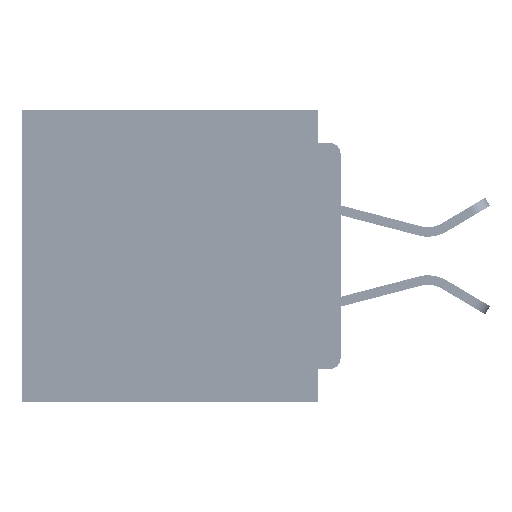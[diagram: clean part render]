
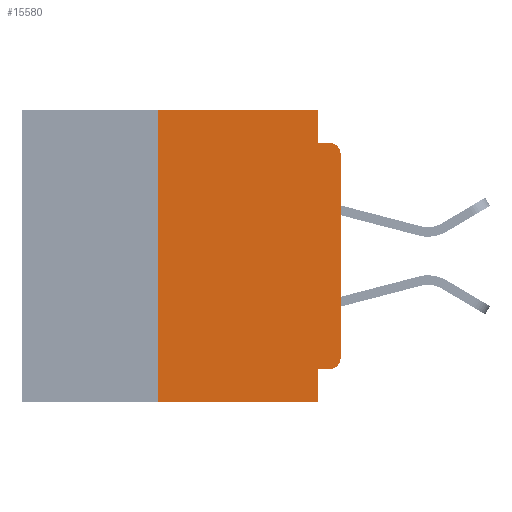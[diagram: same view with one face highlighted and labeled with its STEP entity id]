
A CAD part, left-side view. The second image highlights one B-rep face of the part: STEP entity #15580.
In plain terms, the highlighted planar face has unit normal (-1, 0, 0).
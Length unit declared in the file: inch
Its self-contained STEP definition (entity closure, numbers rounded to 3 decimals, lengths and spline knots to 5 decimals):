
#368 = LINE ( 'NONE', #5651, #32246 ) ;
#454 = ORIENTED_EDGE ( 'NONE', *, *, #24105, .F. ) ;
#1129 = VECTOR ( 'NONE', #30688, 39.37008 ) ;
#1462 = DIRECTION ( 'NONE',  ( 0., 0., 1. ) ) ;
#2603 = VERTEX_POINT ( 'NONE', #30945 ) ;
#2815 = DIRECTION ( 'NONE',  ( -1., 0., 0. ) ) ;
#2857 = CARTESIAN_POINT ( 'NONE',  ( 0., 0.031, -0.4 ) ) ;
#4111 = CARTESIAN_POINT ( 'NONE',  ( 0., 0.015, -0.34 ) ) ;
#5029 = VECTOR ( 'NONE', #46792, 39.37008 ) ;
#5651 = CARTESIAN_POINT ( 'NONE',  ( 0., 0.25, -0.4 ) ) ;
#6347 = AXIS2_PLACEMENT_3D ( 'NONE', #6583, #43711, #19190 ) ;
#6428 = VECTOR ( 'NONE', #40289, 39.37008 ) ;
#6542 = CIRCLE ( 'NONE', #32352, 0.015 ) ;
#6583 = CARTESIAN_POINT ( 'NONE',  ( 0., 0.437, 0. ) ) ;
#6771 = EDGE_CURVE ( 'NONE', #16942, #22062, #12229, .T. ) ;
#7743 = LINE ( 'NONE', #36195, #6428 ) ;
#8335 = DIRECTION ( 'NONE',  ( 0., 0., -1. ) ) ;
#8423 = VECTOR ( 'NONE', #39313, 39.37008 ) ;
#10435 = VERTEX_POINT ( 'NONE', #18213 ) ;
#11214 = ORIENTED_EDGE ( 'NONE', *, *, #42996, .F. ) ;
#11291 = VERTEX_POINT ( 'NONE', #29713 ) ;
#11349 = EDGE_LOOP ( 'NONE', ( #47707, #45500, #45389, #22272, #454, #45478, #36152, #11214, #20267, #26245 ) ) ;
#11424 = EDGE_CURVE ( 'NONE', #2603, #27296, #368, .T. ) ;
#12229 = LINE ( 'NONE', #46842, #1129 ) ;
#13154 = VECTOR ( 'NONE', #25695, 39.37008 ) ;
#13335 = AXIS2_PLACEMENT_3D ( 'NONE', #4111, #33204, #8335 ) ;
#14532 = EDGE_CURVE ( 'NONE', #16942, #49784, #34449, .T. ) ;
#14732 = VERTEX_POINT ( 'NONE', #38306 ) ;
#14991 = PLANE ( 'NONE',  #6347 ) ;
#15276 = VECTOR ( 'NONE', #51262, 39.37008 ) ;
#15580 = ADVANCED_FACE ( 'NONE', ( #29961 ), #14991, .F. ) ;
#16942 = VERTEX_POINT ( 'NONE', #30151 ) ;
#17388 = CARTESIAN_POINT ( 'NONE',  ( 0., 0., -0.06 ) ) ;
#17584 = EDGE_CURVE ( 'NONE', #10435, #14732, #38056, .T. ) ;
#18213 = CARTESIAN_POINT ( 'NONE',  ( 0., 0.031, 0. ) ) ;
#18711 = CARTESIAN_POINT ( 'NONE',  ( 0., 0.031, -0.355 ) ) ;
#18845 = CARTESIAN_POINT ( 'NONE',  ( 0., 0.437, -0.4 ) ) ;
#19152 = CARTESIAN_POINT ( 'NONE',  ( 0., 0., 0. ) ) ;
#19190 = DIRECTION ( 'NONE',  ( 0., 0., -1. ) ) ;
#19510 = EDGE_CURVE ( 'NONE', #14732, #11291, #26344, .T. ) ;
#20267 = ORIENTED_EDGE ( 'NONE', *, *, #6771, .F. ) ;
#22062 = VERTEX_POINT ( 'NONE', #18711 ) ;
#22272 = ORIENTED_EDGE ( 'NONE', *, *, #17584, .F. ) ;
#23401 = VERTEX_POINT ( 'NONE', #17388 ) ;
#24105 = EDGE_CURVE ( 'NONE', #27296, #10435, #43347, .T. ) ;
#24216 = CARTESIAN_POINT ( 'NONE',  ( 0., 0.25, 0. ) ) ;
#25695 = DIRECTION ( 'NONE',  ( 0., -1., 0. ) ) ;
#26245 = ORIENTED_EDGE ( 'NONE', *, *, #14532, .T. ) ;
#26344 = LINE ( 'NONE', #47114, #15276 ) ;
#27231 = LINE ( 'NONE', #19152, #46341 ) ;
#27239 = VERTEX_POINT ( 'NONE', #2857 ) ;
#27296 = VERTEX_POINT ( 'NONE', #24216 ) ;
#27307 = DIRECTION ( 'NONE',  ( 0., 0., 1. ) ) ;
#27789 = CARTESIAN_POINT ( 'NONE',  ( 0., 0.015, -0.06 ) ) ;
#29713 = CARTESIAN_POINT ( 'NONE',  ( 0., 0.015, -0.045 ) ) ;
#29961 = FACE_OUTER_BOUND ( 'NONE', #11349, .T. ) ;
#30151 = CARTESIAN_POINT ( 'NONE',  ( 0., 0.015, -0.355 ) ) ;
#30688 = DIRECTION ( 'NONE',  ( 0., 1., 0. ) ) ;
#30945 = CARTESIAN_POINT ( 'NONE',  ( 0., 0.25, -0.4 ) ) ;
#31912 = DIRECTION ( 'NONE',  ( 0., 0., -1. ) ) ;
#32246 = VECTOR ( 'NONE', #1462, 39.37008 ) ;
#32352 = AXIS2_PLACEMENT_3D ( 'NONE', #27789, #2815, #31912 ) ;
#33127 = LINE ( 'NONE', #18845, #8423 ) ;
#33204 = DIRECTION ( 'NONE',  ( -1., 0., 0. ) ) ;
#34449 = CIRCLE ( 'NONE', #13335, 0.015 ) ;
#36152 = ORIENTED_EDGE ( 'NONE', *, *, #49778, .T. ) ;
#36195 = CARTESIAN_POINT ( 'NONE',  ( 0., 0.031, -0.4 ) ) ;
#38056 = LINE ( 'NONE', #42673, #5029 ) ;
#38306 = CARTESIAN_POINT ( 'NONE',  ( 0., 0.031, -0.045 ) ) ;
#39313 = DIRECTION ( 'NONE',  ( 0., -1., 0. ) ) ;
#40289 = DIRECTION ( 'NONE',  ( 0., 0., -1. ) ) ;
#42153 = EDGE_CURVE ( 'NONE', #23401, #11291, #6542, .T. ) ;
#42673 = CARTESIAN_POINT ( 'NONE',  ( 0., 0.031, 0. ) ) ;
#42996 = EDGE_CURVE ( 'NONE', #22062, #27239, #7743, .T. ) ;
#43347 = LINE ( 'NONE', #46146, #13154 ) ;
#43711 = DIRECTION ( 'NONE',  ( 1., 0., 0. ) ) ;
#45389 = ORIENTED_EDGE ( 'NONE', *, *, #19510, .F. ) ;
#45478 = ORIENTED_EDGE ( 'NONE', *, *, #11424, .F. ) ;
#45500 = ORIENTED_EDGE ( 'NONE', *, *, #42153, .T. ) ;
#46146 = CARTESIAN_POINT ( 'NONE',  ( 0., 0.437, 0. ) ) ;
#46341 = VECTOR ( 'NONE', #27307, 39.37008 ) ;
#46792 = DIRECTION ( 'NONE',  ( 0., 0., -1. ) ) ;
#46842 = CARTESIAN_POINT ( 'NONE',  ( 0., 0., -0.355 ) ) ;
#47114 = CARTESIAN_POINT ( 'NONE',  ( 0., 0., -0.045 ) ) ;
#47311 = CARTESIAN_POINT ( 'NONE',  ( 0., 0., -0.34 ) ) ;
#47707 = ORIENTED_EDGE ( 'NONE', *, *, #50510, .T. ) ;
#49778 = EDGE_CURVE ( 'NONE', #2603, #27239, #33127, .T. ) ;
#49784 = VERTEX_POINT ( 'NONE', #47311 ) ;
#50510 = EDGE_CURVE ( 'NONE', #49784, #23401, #27231, .T. ) ;
#51262 = DIRECTION ( 'NONE',  ( 0., -1., 0. ) ) ;
